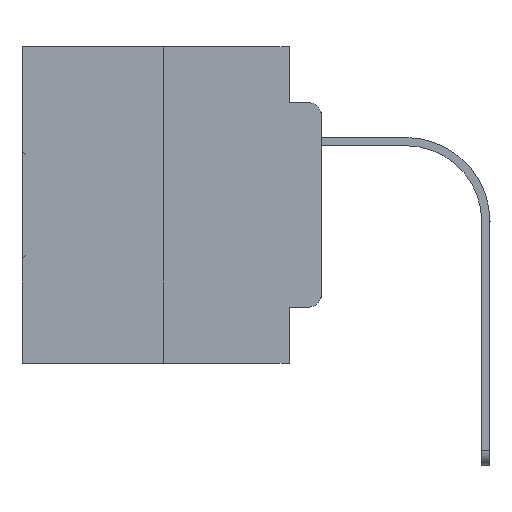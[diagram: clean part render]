
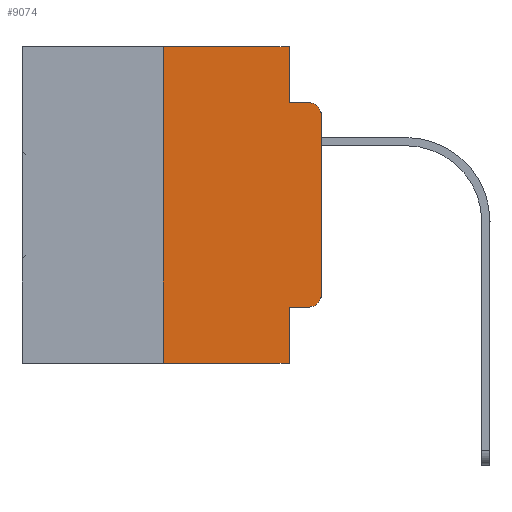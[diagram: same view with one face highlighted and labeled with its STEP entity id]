
A CAD part, left-side view. The second image highlights one B-rep face of the part: STEP entity #9074.
In plain terms, the highlighted planar face has unit normal (-1, 0, 0).
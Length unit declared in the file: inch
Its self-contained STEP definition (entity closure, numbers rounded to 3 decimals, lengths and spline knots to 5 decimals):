
#535 = CARTESIAN_POINT ( 'NONE',  ( 0., 0.02, -0.0885 ) ) ;
#735 = CARTESIAN_POINT ( 'NONE',  ( 0., 0.051, 0. ) ) ;
#1114 = CARTESIAN_POINT ( 'NONE',  ( 0., 0.051, 0. ) ) ;
#1571 = CARTESIAN_POINT ( 'NONE',  ( 0., 0.25, 0. ) ) ;
#2134 = EDGE_CURVE ( 'NONE', #19734, #18269, #31511, .T. ) ;
#2223 = ORIENTED_EDGE ( 'NONE', *, *, #24478, .F. ) ;
#3580 = DIRECTION ( 'NONE',  ( 0., 0., -1. ) ) ;
#3971 = CARTESIAN_POINT ( 'NONE',  ( 0., 0.473, 0. ) ) ;
#4197 = ORIENTED_EDGE ( 'NONE', *, *, #9133, .T. ) ;
#6340 = VERTEX_POINT ( 'NONE', #23784 ) ;
#6378 = CARTESIAN_POINT ( 'NONE',  ( 0., 0.473, 0. ) ) ;
#6405 = DIRECTION ( 'NONE',  ( 1., 0., 0. ) ) ;
#6411 = CARTESIAN_POINT ( 'NONE',  ( 0., 0.051, -0.0885 ) ) ;
#6641 = VECTOR ( 'NONE', #10696, 39.37008 ) ;
#6905 = ORIENTED_EDGE ( 'NONE', *, *, #21602, .F. ) ;
#7216 = EDGE_CURVE ( 'NONE', #11925, #18269, #13130, .T. ) ;
#7266 = DIRECTION ( 'NONE',  ( 0., -1., 0. ) ) ;
#8113 = LINE ( 'NONE', #1114, #18588 ) ;
#8454 = CARTESIAN_POINT ( 'NONE',  ( 0., 0.02, -0.1085 ) ) ;
#8599 = DIRECTION ( 'NONE',  ( 0., 0., 1. ) ) ;
#8676 = DIRECTION ( 'NONE',  ( 0., -1., 0. ) ) ;
#8915 = LINE ( 'NONE', #21110, #26558 ) ;
#9017 = VECTOR ( 'NONE', #21210, 39.37008 ) ;
#9074 = ADVANCED_FACE ( 'NONE', ( #30656 ), #18794, .F. ) ;
#9133 = EDGE_CURVE ( 'NONE', #11925, #13034, #13752, .T. ) ;
#9163 = ORIENTED_EDGE ( 'NONE', *, *, #23987, .T. ) ;
#9234 = ORIENTED_EDGE ( 'NONE', *, *, #25145, .T. ) ;
#10696 = DIRECTION ( 'NONE',  ( 0., 0., -1. ) ) ;
#11021 = CARTESIAN_POINT ( 'NONE',  ( 0., 0.02, -0.3915 ) ) ;
#11115 = LINE ( 'NONE', #6378, #19913 ) ;
#11899 = CARTESIAN_POINT ( 'NONE',  ( 0., 0.02, -0.4115 ) ) ;
#11925 = VERTEX_POINT ( 'NONE', #21468 ) ;
#12001 = VERTEX_POINT ( 'NONE', #19363 ) ;
#12935 = AXIS2_PLACEMENT_3D ( 'NONE', #8454, #27986, #3580 ) ;
#13007 = DIRECTION ( 'NONE',  ( 0., 0., -1. ) ) ;
#13034 = VERTEX_POINT ( 'NONE', #11899 ) ;
#13130 = LINE ( 'NONE', #28096, #6641 ) ;
#13752 = LINE ( 'NONE', #23657, #9017 ) ;
#14908 = EDGE_LOOP ( 'NONE', ( #28242, #9234, #2223, #19423, #25320, #6905, #15526, #24724, #4197, #9163 ) ) ;
#15054 = VERTEX_POINT ( 'NONE', #1571 ) ;
#15240 = VECTOR ( 'NONE', #7266, 39.37008 ) ;
#15526 = ORIENTED_EDGE ( 'NONE', *, *, #2134, .T. ) ;
#15632 = VECTOR ( 'NONE', #24593, 39.37008 ) ;
#16563 = VECTOR ( 'NONE', #29026, 39.37008 ) ;
#17832 = AXIS2_PLACEMENT_3D ( 'NONE', #3971, #6405, #21368 ) ;
#18269 = VERTEX_POINT ( 'NONE', #27293 ) ;
#18507 = DIRECTION ( 'NONE',  ( -1., 0., 0. ) ) ;
#18588 = VECTOR ( 'NONE', #13007, 39.37008 ) ;
#18617 = CIRCLE ( 'NONE', #22213, 0.02 ) ;
#18794 = PLANE ( 'NONE',  #17832 ) ;
#19363 = CARTESIAN_POINT ( 'NONE',  ( 0., 0.051, -0.0885 ) ) ;
#19423 = ORIENTED_EDGE ( 'NONE', *, *, #28353, .F. ) ;
#19564 = CARTESIAN_POINT ( 'NONE',  ( 0., 0., 0. ) ) ;
#19734 = VERTEX_POINT ( 'NONE', #30542 ) ;
#19913 = VECTOR ( 'NONE', #8676, 39.37008 ) ;
#21005 = EDGE_CURVE ( 'NONE', #24667, #6340, #21835, .T. ) ;
#21110 = CARTESIAN_POINT ( 'NONE',  ( 0., 0.25, 0. ) ) ;
#21210 = DIRECTION ( 'NONE',  ( 0., -1., 0. ) ) ;
#21368 = DIRECTION ( 'NONE',  ( 0., 0., -1. ) ) ;
#21373 = LINE ( 'NONE', #6411, #16563 ) ;
#21468 = CARTESIAN_POINT ( 'NONE',  ( 0., 0.051, -0.4115 ) ) ;
#21602 = EDGE_CURVE ( 'NONE', #19734, #15054, #8915, .T. ) ;
#21835 = LINE ( 'NONE', #19564, #15632 ) ;
#22069 = CARTESIAN_POINT ( 'NONE',  ( 0., 0.473, -0.5 ) ) ;
#22213 = AXIS2_PLACEMENT_3D ( 'NONE', #11021, #18507, #28415 ) ;
#22788 = CIRCLE ( 'NONE', #12935, 0.02 ) ;
#23657 = CARTESIAN_POINT ( 'NONE',  ( 0., 0.051, -0.4115 ) ) ;
#23784 = CARTESIAN_POINT ( 'NONE',  ( 0., 0., -0.1085 ) ) ;
#23987 = EDGE_CURVE ( 'NONE', #13034, #24667, #18617, .T. ) ;
#24478 = EDGE_CURVE ( 'NONE', #12001, #30866, #21373, .T. ) ;
#24593 = DIRECTION ( 'NONE',  ( 0., 0., 1. ) ) ;
#24667 = VERTEX_POINT ( 'NONE', #29973 ) ;
#24724 = ORIENTED_EDGE ( 'NONE', *, *, #7216, .F. ) ;
#25145 = EDGE_CURVE ( 'NONE', #6340, #30866, #22788, .T. ) ;
#25320 = ORIENTED_EDGE ( 'NONE', *, *, #27310, .F. ) ;
#25573 = VERTEX_POINT ( 'NONE', #735 ) ;
#26558 = VECTOR ( 'NONE', #8599, 39.37008 ) ;
#27293 = CARTESIAN_POINT ( 'NONE',  ( 0., 0.051, -0.5 ) ) ;
#27310 = EDGE_CURVE ( 'NONE', #15054, #25573, #11115, .T. ) ;
#27986 = DIRECTION ( 'NONE',  ( -1., 0., 0. ) ) ;
#28096 = CARTESIAN_POINT ( 'NONE',  ( 0., 0.051, 0. ) ) ;
#28242 = ORIENTED_EDGE ( 'NONE', *, *, #21005, .T. ) ;
#28353 = EDGE_CURVE ( 'NONE', #25573, #12001, #8113, .T. ) ;
#28415 = DIRECTION ( 'NONE',  ( 0., 0., -1. ) ) ;
#29026 = DIRECTION ( 'NONE',  ( 0., -1., 0. ) ) ;
#29973 = CARTESIAN_POINT ( 'NONE',  ( 0., 0., -0.3915 ) ) ;
#30542 = CARTESIAN_POINT ( 'NONE',  ( 0., 0.25, -0.5 ) ) ;
#30656 = FACE_OUTER_BOUND ( 'NONE', #14908, .T. ) ;
#30866 = VERTEX_POINT ( 'NONE', #535 ) ;
#31511 = LINE ( 'NONE', #22069, #15240 ) ;
